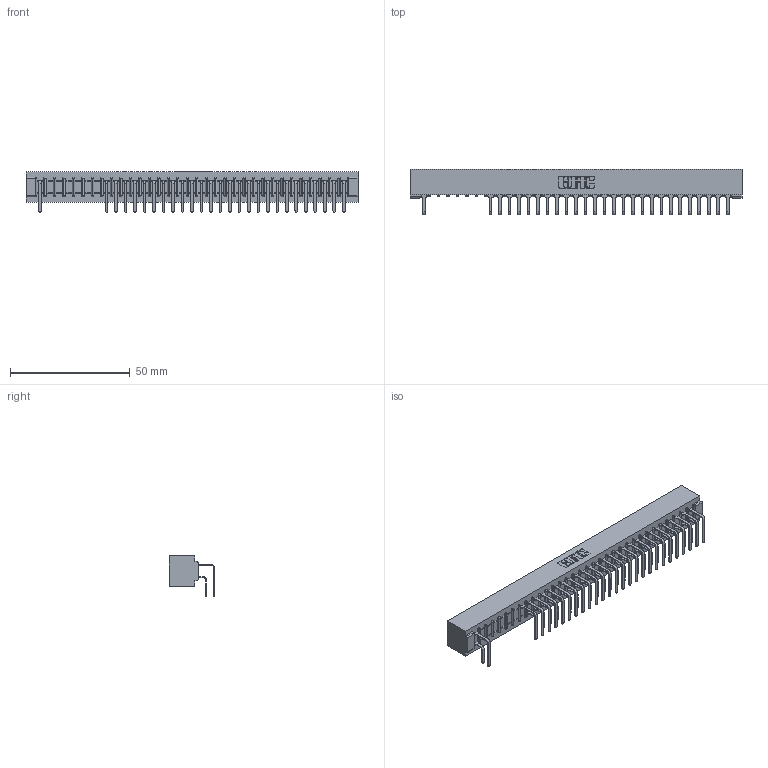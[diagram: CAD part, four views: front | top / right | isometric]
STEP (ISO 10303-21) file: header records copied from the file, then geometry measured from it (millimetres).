
FILE_DESCRIPTION (( 'STEP AP203' ), '1' );
FILE_NAME ('307-033-558-101.STEP', '2018-08-04T23:33:59', ( '' ), ( '' ), 'SwSTEP 2.0', 'SolidWorks 2016', '' );
FILE_SCHEMA (( 'CONFIG_CONTROL_DESIGN' ));
Length unit declared in the file: inch
Products named in the file (4): 307 Part_No Mounting Lugs; 307-290-001_558 559 - 1 (Single); 307-290-001_558 - 2 (Single); 307-033-558-101
Assembly tree (54 placements, depth 2):
  307-033-558-101
    307 Part_No Mounting Lugs
    307-290-001_558 559 - 1 (Single)  x26
    307-290-001_558 - 2 (Single)  x27
Bounding box: 138.63 x 18.96 x 16.8 mm (x, y, z)
Volume: 15294.1 mm3; surface area: 19120.8 mm2
Topology: 54 solids, 54 shells, 2924 faces, 8241 edges, 5330 vertices
Faces by surface type: plane 1893, cylinder 963, sphere 68
Entity records: 31209 total; most frequent: CARTESIAN_POINT 5162, ORIENTED_EDGE 5126, DIRECTION 5045, EDGE_CURVE 2563, VECTOR 1963, LINE 1963, VERTEX_POINT 1658, AXIS2_PLACEMENT_3D 1541
